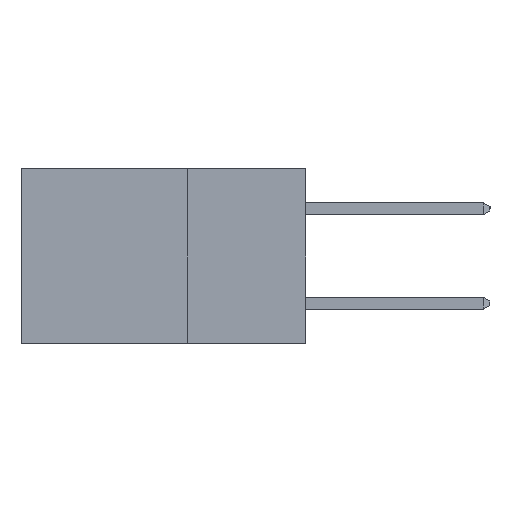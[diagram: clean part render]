
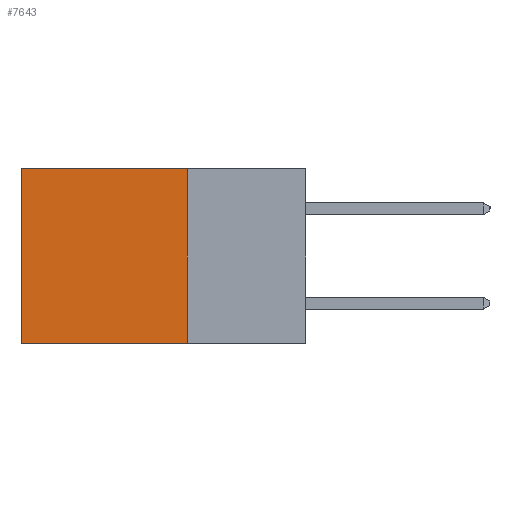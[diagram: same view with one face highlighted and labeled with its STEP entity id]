
A CAD part, left-side view. The second image highlights one B-rep face of the part: STEP entity #7643.
In plain terms, the highlighted planar face has unit normal (-1, 0, 0).
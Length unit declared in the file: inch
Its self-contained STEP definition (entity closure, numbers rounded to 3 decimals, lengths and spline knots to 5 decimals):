
#340 = DIRECTION ( 'NONE',  ( 0., 0., -1. ) ) ;
#571 = FACE_OUTER_BOUND ( 'NONE', #4097, .T. ) ;
#1132 = DIRECTION ( 'NONE',  ( 0., 1., 0. ) ) ;
#1659 = EDGE_CURVE ( 'NONE', #8377, #8147, #5608, .T. ) ;
#2220 = DIRECTION ( 'NONE',  ( 1., 0., 0. ) ) ;
#2414 = CARTESIAN_POINT ( 'NONE',  ( 0.2615, 0.6, -0.37 ) ) ;
#2994 = DIRECTION ( 'NONE',  ( 0., 0., -1. ) ) ;
#3002 = CARTESIAN_POINT ( 'NONE',  ( 0.2615, 0.6, -0.37 ) ) ;
#3118 = LINE ( 'NONE', #7585, #6338 ) ;
#3946 = EDGE_CURVE ( 'NONE', #8147, #7149, #8485, .T. ) ;
#4002 = DIRECTION ( 'NONE',  ( 0., 1., 0. ) ) ;
#4097 = EDGE_LOOP ( 'NONE', ( #7391, #6760, #6382, #10377 ) ) ;
#4884 = PLANE ( 'NONE',  #11277 ) ;
#5417 = LINE ( 'NONE', #10895, #11244 ) ;
#5608 = LINE ( 'NONE', #9206, #7209 ) ;
#5803 = CARTESIAN_POINT ( 'NONE',  ( 0.2615, 0.25, -0.37 ) ) ;
#5876 = EDGE_CURVE ( 'NONE', #6492, #7149, #3118, .T. ) ;
#6338 = VECTOR ( 'NONE', #4002, 39.37008 ) ;
#6382 = ORIENTED_EDGE ( 'NONE', *, *, #7538, .F. ) ;
#6492 = VERTEX_POINT ( 'NONE', #5803 ) ;
#6566 = CARTESIAN_POINT ( 'NONE',  ( 0.2615, 0.6, 0. ) ) ;
#6760 = ORIENTED_EDGE ( 'NONE', *, *, #5876, .F. ) ;
#7149 = VERTEX_POINT ( 'NONE', #2414 ) ;
#7209 = VECTOR ( 'NONE', #1132, 39.37008 ) ;
#7391 = ORIENTED_EDGE ( 'NONE', *, *, #3946, .T. ) ;
#7538 = EDGE_CURVE ( 'NONE', #8377, #6492, #5417, .T. ) ;
#7585 = CARTESIAN_POINT ( 'NONE',  ( 0.2615, 0.25, -0.37 ) ) ;
#7643 = ADVANCED_FACE ( 'NONE', ( #571 ), #4884, .F. ) ;
#8147 = VERTEX_POINT ( 'NONE', #6566 ) ;
#8377 = VERTEX_POINT ( 'NONE', #9241 ) ;
#8477 = CARTESIAN_POINT ( 'NONE',  ( 0.2615, 0.25, -0.37 ) ) ;
#8485 = LINE ( 'NONE', #3002, #10263 ) ;
#9206 = CARTESIAN_POINT ( 'NONE',  ( 0.2615, 0.25, 0. ) ) ;
#9241 = CARTESIAN_POINT ( 'NONE',  ( 0.2615, 0.25, 0. ) ) ;
#10246 = DIRECTION ( 'NONE',  ( 0., 0., -1. ) ) ;
#10263 = VECTOR ( 'NONE', #10246, 39.37008 ) ;
#10377 = ORIENTED_EDGE ( 'NONE', *, *, #1659, .T. ) ;
#10895 = CARTESIAN_POINT ( 'NONE',  ( 0.2615, 0.25, -0.37 ) ) ;
#11244 = VECTOR ( 'NONE', #2994, 39.37008 ) ;
#11277 = AXIS2_PLACEMENT_3D ( 'NONE', #8477, #2220, #340 ) ;
